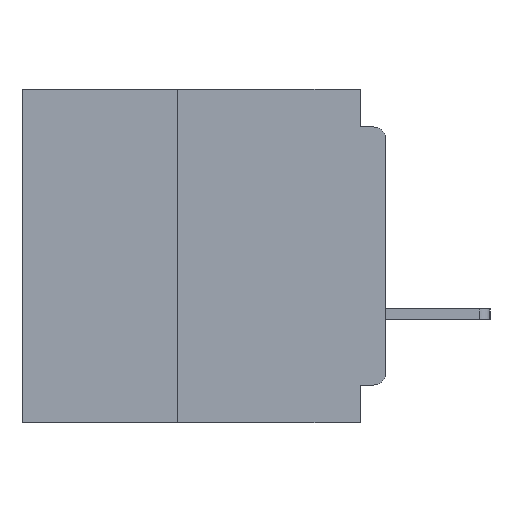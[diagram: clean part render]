
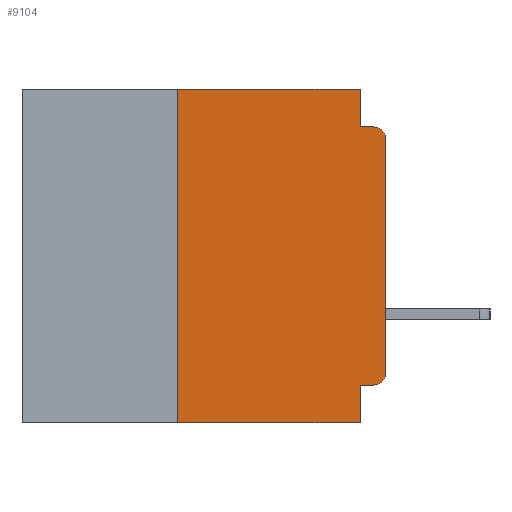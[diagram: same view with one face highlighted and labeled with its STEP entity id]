
A CAD part, left-side view. The second image highlights one B-rep face of the part: STEP entity #9104.
In plain terms, the highlighted planar face has unit normal (-1, 0, 0).
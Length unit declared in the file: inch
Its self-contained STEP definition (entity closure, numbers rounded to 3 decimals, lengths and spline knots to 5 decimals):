
#965 = VECTOR ( 'NONE', #19598, 39.37008 ) ;
#1284 = EDGE_CURVE ( 'NONE', #27278, #55175, #36976, .T. ) ;
#2807 = DIRECTION ( 'NONE',  ( 1., 0., 0. ) ) ;
#2945 = LINE ( 'NONE', #37625, #53227 ) ;
#3037 = AXIS2_PLACEMENT_3D ( 'NONE', #45734, #16564, #50624 ) ;
#3268 = EDGE_LOOP ( 'NONE', ( #7950, #47790, #35572, #53360, #24522, #9245, #18437, #55936, #62909, #19735 ) ) ;
#3816 = DIRECTION ( 'NONE',  ( 0., 0., -1. ) ) ;
#4565 = AXIS2_PLACEMENT_3D ( 'NONE', #31979, #2807, #36886 ) ;
#4936 = CARTESIAN_POINT ( 'NONE',  ( 0., 0., -0.06 ) ) ;
#5612 = VECTOR ( 'NONE', #54223, 39.37008 ) ;
#7950 = ORIENTED_EDGE ( 'NONE', *, *, #62887, .T. ) ;
#9104 = ADVANCED_FACE ( 'NONE', ( #33829 ), #17268, .F. ) ;
#9245 = ORIENTED_EDGE ( 'NONE', *, *, #40081, .F. ) ;
#11696 = DIRECTION ( 'NONE',  ( 0., 0., 1. ) ) ;
#13356 = CARTESIAN_POINT ( 'NONE',  ( 0., 0.015, -0.06 ) ) ;
#15109 = EDGE_CURVE ( 'NONE', #27278, #20127, #2945, .T. ) ;
#15517 = CIRCLE ( 'NONE', #24046, 0.015 ) ;
#16564 = DIRECTION ( 'NONE',  ( -1., 0., 0. ) ) ;
#17268 = PLANE ( 'NONE',  #4565 ) ;
#17773 = VERTEX_POINT ( 'NONE', #35533 ) ;
#18225 = DIRECTION ( 'NONE',  ( 0., 0., -1. ) ) ;
#18437 = ORIENTED_EDGE ( 'NONE', *, *, #54875, .T. ) ;
#19598 = DIRECTION ( 'NONE',  ( 0., 0., -1. ) ) ;
#19735 = ORIENTED_EDGE ( 'NONE', *, *, #1284, .T. ) ;
#20127 = VERTEX_POINT ( 'NONE', #26788 ) ;
#23207 = LINE ( 'NONE', #47585, #50610 ) ;
#23328 = DIRECTION ( 'NONE',  ( 0., -1., 0. ) ) ;
#23596 = CARTESIAN_POINT ( 'NONE',  ( 0., 0.015, -0.045 ) ) ;
#24046 = AXIS2_PLACEMENT_3D ( 'NONE', #13356, #47402, #18225 ) ;
#24522 = ORIENTED_EDGE ( 'NONE', *, *, #28905, .F. ) ;
#25064 = VECTOR ( 'NONE', #25282, 39.37008 ) ;
#25083 = CARTESIAN_POINT ( 'NONE',  ( 0., 0.437, 0. ) ) ;
#25282 = DIRECTION ( 'NONE',  ( 0., 0., 1. ) ) ;
#26788 = CARTESIAN_POINT ( 'NONE',  ( 0., 0.031, -0.355 ) ) ;
#27278 = VERTEX_POINT ( 'NONE', #28569 ) ;
#27356 = VERTEX_POINT ( 'NONE', #4936 ) ;
#27359 = LINE ( 'NONE', #28077, #28896 ) ;
#28077 = CARTESIAN_POINT ( 'NONE',  ( 0., 0.031, -0.4 ) ) ;
#28421 = EDGE_CURVE ( 'NONE', #60741, #46970, #23207, .T. ) ;
#28569 = CARTESIAN_POINT ( 'NONE',  ( 0., 0.015, -0.355 ) ) ;
#28896 = VECTOR ( 'NONE', #3816, 39.37008 ) ;
#28905 = EDGE_CURVE ( 'NONE', #46759, #17773, #42941, .T. ) ;
#29969 = CARTESIAN_POINT ( 'NONE',  ( 0., 0., 0. ) ) ;
#30088 = EDGE_CURVE ( 'NONE', #17773, #60741, #38289, .T. ) ;
#31979 = CARTESIAN_POINT ( 'NONE',  ( 0., 0.437, 0. ) ) ;
#33829 = FACE_OUTER_BOUND ( 'NONE', #3268, .T. ) ;
#35533 = CARTESIAN_POINT ( 'NONE',  ( 0., 0.031, 0. ) ) ;
#35572 = ORIENTED_EDGE ( 'NONE', *, *, #28421, .F. ) ;
#36886 = DIRECTION ( 'NONE',  ( 0., 0., -1. ) ) ;
#36976 = CIRCLE ( 'NONE', #3037, 0.015 ) ;
#37625 = CARTESIAN_POINT ( 'NONE',  ( 0., 0., -0.355 ) ) ;
#38015 = LINE ( 'NONE', #29969, #25064 ) ;
#38130 = VECTOR ( 'NONE', #11696, 39.37008 ) ;
#38289 = LINE ( 'NONE', #48785, #965 ) ;
#40081 = EDGE_CURVE ( 'NONE', #53063, #46759, #48007, .T. ) ;
#40843 = CARTESIAN_POINT ( 'NONE',  ( 0., 0.25, -0.4 ) ) ;
#41297 = CARTESIAN_POINT ( 'NONE',  ( 0., 0.25, 0. ) ) ;
#41837 = VERTEX_POINT ( 'NONE', #58897 ) ;
#42941 = LINE ( 'NONE', #25083, #5612 ) ;
#44503 = CARTESIAN_POINT ( 'NONE',  ( 0., 0., -0.34 ) ) ;
#45734 = CARTESIAN_POINT ( 'NONE',  ( 0., 0.015, -0.34 ) ) ;
#46759 = VERTEX_POINT ( 'NONE', #41297 ) ;
#46883 = CARTESIAN_POINT ( 'NONE',  ( 0., 0.437, -0.4 ) ) ;
#46970 = VERTEX_POINT ( 'NONE', #23596 ) ;
#47402 = DIRECTION ( 'NONE',  ( -1., 0., 0. ) ) ;
#47585 = CARTESIAN_POINT ( 'NONE',  ( 0., 0., -0.045 ) ) ;
#47790 = ORIENTED_EDGE ( 'NONE', *, *, #60311, .T. ) ;
#47939 = VECTOR ( 'NONE', #61510, 39.37008 ) ;
#48007 = LINE ( 'NONE', #40843, #38130 ) ;
#48785 = CARTESIAN_POINT ( 'NONE',  ( 0., 0.031, 0. ) ) ;
#50610 = VECTOR ( 'NONE', #23328, 39.37008 ) ;
#50624 = DIRECTION ( 'NONE',  ( 0., 0., -1. ) ) ;
#53063 = VERTEX_POINT ( 'NONE', #62775 ) ;
#53227 = VECTOR ( 'NONE', #56969, 39.37008 ) ;
#53360 = ORIENTED_EDGE ( 'NONE', *, *, #30088, .F. ) ;
#54223 = DIRECTION ( 'NONE',  ( 0., -1., 0. ) ) ;
#54875 = EDGE_CURVE ( 'NONE', #53063, #41837, #60829, .T. ) ;
#55175 = VERTEX_POINT ( 'NONE', #44503 ) ;
#55650 = CARTESIAN_POINT ( 'NONE',  ( 0., 0.031, -0.045 ) ) ;
#55936 = ORIENTED_EDGE ( 'NONE', *, *, #62651, .F. ) ;
#56969 = DIRECTION ( 'NONE',  ( 0., 1., 0. ) ) ;
#58897 = CARTESIAN_POINT ( 'NONE',  ( 0., 0.031, -0.4 ) ) ;
#60311 = EDGE_CURVE ( 'NONE', #27356, #46970, #15517, .T. ) ;
#60741 = VERTEX_POINT ( 'NONE', #55650 ) ;
#60829 = LINE ( 'NONE', #46883, #47939 ) ;
#61510 = DIRECTION ( 'NONE',  ( 0., -1., 0. ) ) ;
#62651 = EDGE_CURVE ( 'NONE', #20127, #41837, #27359, .T. ) ;
#62775 = CARTESIAN_POINT ( 'NONE',  ( 0., 0.25, -0.4 ) ) ;
#62887 = EDGE_CURVE ( 'NONE', #55175, #27356, #38015, .T. ) ;
#62909 = ORIENTED_EDGE ( 'NONE', *, *, #15109, .F. ) ;
